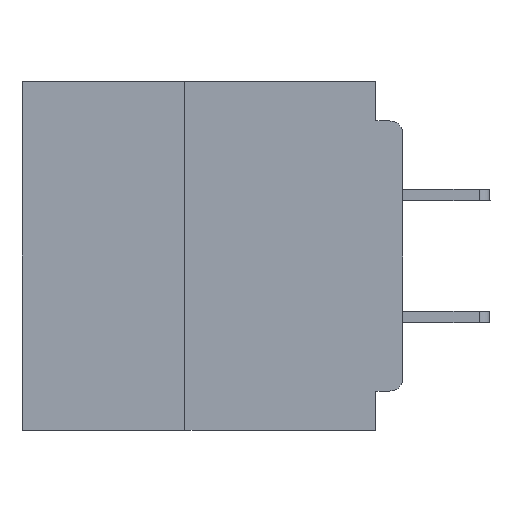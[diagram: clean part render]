
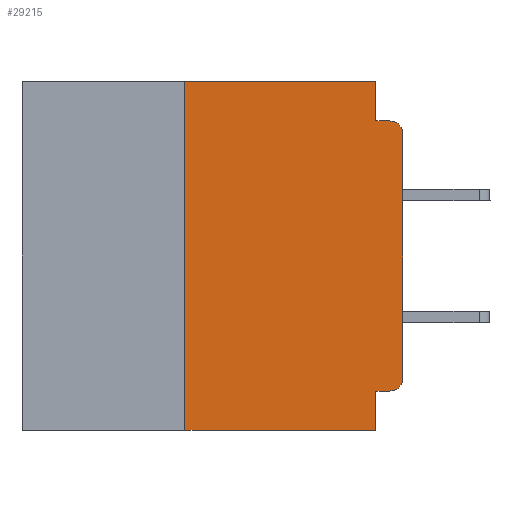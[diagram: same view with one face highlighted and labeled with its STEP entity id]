
A CAD part, left-side view. The second image highlights one B-rep face of the part: STEP entity #29215.
In plain terms, the highlighted planar face has unit normal (-1, 0, 0).
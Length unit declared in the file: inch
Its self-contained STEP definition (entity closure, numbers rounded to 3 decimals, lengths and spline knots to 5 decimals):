
#106 = ORIENTED_EDGE ( 'NONE', *, *, #38779, .F. ) ;
#1104 = CIRCLE ( 'NONE', #25393, 0.015 ) ;
#1456 = ORIENTED_EDGE ( 'NONE', *, *, #17696, .F. ) ;
#1871 = CARTESIAN_POINT ( 'NONE',  ( 0., 0.031, 0. ) ) ;
#2037 = ORIENTED_EDGE ( 'NONE', *, *, #29667, .F. ) ;
#2704 = VECTOR ( 'NONE', #55672, 39.37008 ) ;
#2713 = DIRECTION ( 'NONE',  ( 0., -1., 0. ) ) ;
#3315 = CARTESIAN_POINT ( 'NONE',  ( 0., 0.015, -0.045 ) ) ;
#3363 = LINE ( 'NONE', #47506, #28940 ) ;
#4168 = DIRECTION ( 'NONE',  ( 0., 0., 1. ) ) ;
#4425 = ORIENTED_EDGE ( 'NONE', *, *, #57883, .F. ) ;
#6962 = DIRECTION ( 'NONE',  ( 0., 1., 0. ) ) ;
#7028 = VECTOR ( 'NONE', #12141, 39.37008 ) ;
#8140 = VERTEX_POINT ( 'NONE', #24549 ) ;
#10132 = PLANE ( 'NONE',  #46337 ) ;
#11121 = CARTESIAN_POINT ( 'NONE',  ( 0., 0.015, -0.355 ) ) ;
#11184 = EDGE_CURVE ( 'NONE', #61548, #35685, #52891, .T. ) ;
#11444 = ORIENTED_EDGE ( 'NONE', *, *, #31332, .T. ) ;
#12141 = DIRECTION ( 'NONE',  ( 0., -1., 0. ) ) ;
#12164 = DIRECTION ( 'NONE',  ( -1., 0., 0. ) ) ;
#14757 = CARTESIAN_POINT ( 'NONE',  ( 0., 0.031, -0.355 ) ) ;
#14942 = ORIENTED_EDGE ( 'NONE', *, *, #11184, .F. ) ;
#15482 = CARTESIAN_POINT ( 'NONE',  ( 0., 0.437, 0. ) ) ;
#17696 = EDGE_CURVE ( 'NONE', #21028, #30720, #44470, .T. ) ;
#18378 = VERTEX_POINT ( 'NONE', #27522 ) ;
#18656 = CARTESIAN_POINT ( 'NONE',  ( 0., 0.015, -0.34 ) ) ;
#19434 = CARTESIAN_POINT ( 'NONE',  ( 0., 0.25, -0.4 ) ) ;
#19641 = CIRCLE ( 'NONE', #36234, 0.015 ) ;
#19755 = FACE_OUTER_BOUND ( 'NONE', #26952, .T. ) ;
#19960 = CARTESIAN_POINT ( 'NONE',  ( 0., 0., -0.06 ) ) ;
#20115 = CARTESIAN_POINT ( 'NONE',  ( 0., 0., 0. ) ) ;
#20418 = VERTEX_POINT ( 'NONE', #19960 ) ;
#20614 = DIRECTION ( 'NONE',  ( 1., 0., 0. ) ) ;
#21028 = VERTEX_POINT ( 'NONE', #14757 ) ;
#22948 = CARTESIAN_POINT ( 'NONE',  ( 0., 0.031, -0.4 ) ) ;
#23169 = DIRECTION ( 'NONE',  ( 0., 0., -1. ) ) ;
#23783 = DIRECTION ( 'NONE',  ( 0., 0., -1. ) ) ;
#24549 = CARTESIAN_POINT ( 'NONE',  ( 0., 0.25, -0.4 ) ) ;
#25393 = AXIS2_PLACEMENT_3D ( 'NONE', #42675, #12164, #47767 ) ;
#26952 = EDGE_LOOP ( 'NONE', ( #62782, #36749, #106, #14942, #4425, #2037, #45607, #1456, #36510, #11444 ) ) ;
#27522 = CARTESIAN_POINT ( 'NONE',  ( 0., 0.25, 0. ) ) ;
#28243 = CARTESIAN_POINT ( 'NONE',  ( 0., 0.031, 0. ) ) ;
#28940 = VECTOR ( 'NONE', #6962, 39.37008 ) ;
#29215 = ADVANCED_FACE ( 'NONE', ( #19755 ), #10132, .F. ) ;
#29667 = EDGE_CURVE ( 'NONE', #8140, #18378, #54071, .T. ) ;
#30720 = VERTEX_POINT ( 'NONE', #22948 ) ;
#30873 = VECTOR ( 'NONE', #65484, 39.37008 ) ;
#31332 = EDGE_CURVE ( 'NONE', #42547, #47257, #19641, .T. ) ;
#31507 = LINE ( 'NONE', #20115, #2704 ) ;
#32993 = CARTESIAN_POINT ( 'NONE',  ( 0., 0., -0.34 ) ) ;
#34987 = LINE ( 'NONE', #60475, #60374 ) ;
#35523 = EDGE_CURVE ( 'NONE', #8140, #30720, #34987, .T. ) ;
#35685 = VERTEX_POINT ( 'NONE', #51357 ) ;
#36234 = AXIS2_PLACEMENT_3D ( 'NONE', #18656, #54217, #23783 ) ;
#36510 = ORIENTED_EDGE ( 'NONE', *, *, #47884, .F. ) ;
#36749 = ORIENTED_EDGE ( 'NONE', *, *, #37702, .T. ) ;
#37030 = LINE ( 'NONE', #58696, #45767 ) ;
#37702 = EDGE_CURVE ( 'NONE', #20418, #52765, #1104, .T. ) ;
#37842 = VECTOR ( 'NONE', #23169, 39.37008 ) ;
#38779 = EDGE_CURVE ( 'NONE', #35685, #52765, #37030, .T. ) ;
#40270 = CARTESIAN_POINT ( 'NONE',  ( 0., 0.031, -0.4 ) ) ;
#40585 = VECTOR ( 'NONE', #4168, 39.37008 ) ;
#42547 = VERTEX_POINT ( 'NONE', #11121 ) ;
#42655 = CARTESIAN_POINT ( 'NONE',  ( 0., 0.437, 0. ) ) ;
#42675 = CARTESIAN_POINT ( 'NONE',  ( 0., 0.015, -0.06 ) ) ;
#44470 = LINE ( 'NONE', #40270, #30873 ) ;
#45607 = ORIENTED_EDGE ( 'NONE', *, *, #35523, .T. ) ;
#45767 = VECTOR ( 'NONE', #2713, 39.37008 ) ;
#46337 = AXIS2_PLACEMENT_3D ( 'NONE', #15482, #20614, #56158 ) ;
#47257 = VERTEX_POINT ( 'NONE', #32993 ) ;
#47506 = CARTESIAN_POINT ( 'NONE',  ( 0., 0., -0.355 ) ) ;
#47767 = DIRECTION ( 'NONE',  ( 0., 0., -1. ) ) ;
#47884 = EDGE_CURVE ( 'NONE', #42547, #21028, #3363, .T. ) ;
#51357 = CARTESIAN_POINT ( 'NONE',  ( 0., 0.031, -0.045 ) ) ;
#52765 = VERTEX_POINT ( 'NONE', #3315 ) ;
#52891 = LINE ( 'NONE', #28243, #37842 ) ;
#54071 = LINE ( 'NONE', #19434, #40585 ) ;
#54217 = DIRECTION ( 'NONE',  ( -1., 0., 0. ) ) ;
#55672 = DIRECTION ( 'NONE',  ( 0., 0., 1. ) ) ;
#56158 = DIRECTION ( 'NONE',  ( 0., 0., -1. ) ) ;
#57883 = EDGE_CURVE ( 'NONE', #18378, #61548, #61145, .T. ) ;
#58696 = CARTESIAN_POINT ( 'NONE',  ( 0., 0., -0.045 ) ) ;
#59532 = EDGE_CURVE ( 'NONE', #47257, #20418, #31507, .T. ) ;
#60374 = VECTOR ( 'NONE', #65531, 39.37008 ) ;
#60475 = CARTESIAN_POINT ( 'NONE',  ( 0., 0.437, -0.4 ) ) ;
#61145 = LINE ( 'NONE', #42655, #7028 ) ;
#61548 = VERTEX_POINT ( 'NONE', #1871 ) ;
#62782 = ORIENTED_EDGE ( 'NONE', *, *, #59532, .T. ) ;
#65484 = DIRECTION ( 'NONE',  ( 0., 0., -1. ) ) ;
#65531 = DIRECTION ( 'NONE',  ( 0., -1., 0. ) ) ;
